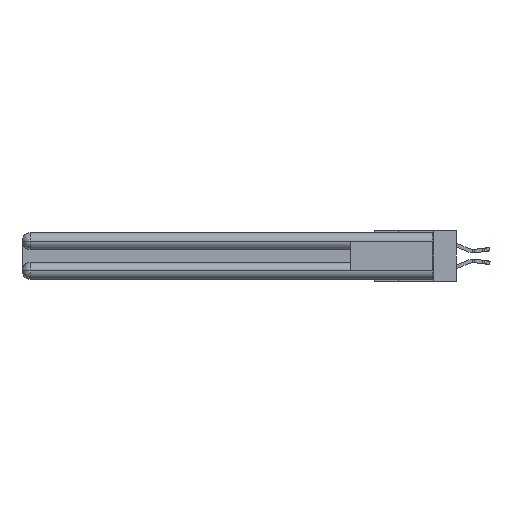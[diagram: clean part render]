
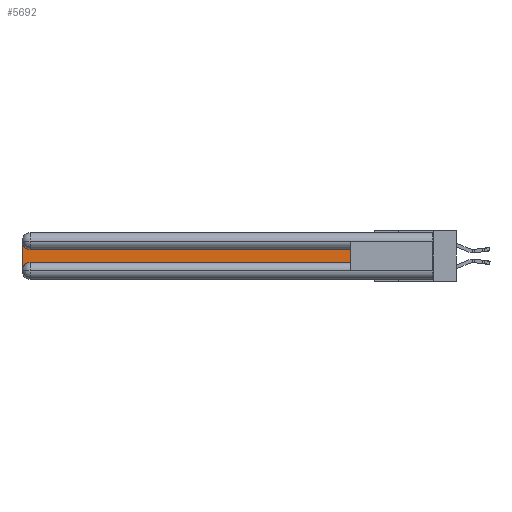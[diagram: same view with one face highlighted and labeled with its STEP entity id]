
A CAD part, left-side view. The second image highlights one B-rep face of the part: STEP entity #5692.
In plain terms, the highlighted planar face has unit normal (-1, 0, 0).
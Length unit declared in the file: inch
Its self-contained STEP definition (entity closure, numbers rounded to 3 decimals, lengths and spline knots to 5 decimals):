
#187 = ORIENTED_EDGE ( 'NONE', *, *, #18927, .T. ) ;
#1337 = VECTOR ( 'NONE', #25625, 39.37008 ) ;
#1376 = CIRCLE ( 'NONE', #27915, 0.06 ) ;
#1756 = AXIS2_PLACEMENT_3D ( 'NONE', #16914, #13825, #24627 ) ;
#2219 = CARTESIAN_POINT ( 'NONE',  ( 0.075, 0.6, -0.2175 ) ) ;
#2345 = CARTESIAN_POINT ( 'NONE',  ( 0.075, 2.94, -0.1225 ) ) ;
#2535 = FACE_OUTER_BOUND ( 'NONE', #12113, .T. ) ;
#2604 = CARTESIAN_POINT ( 'NONE',  ( 0.075, 0.6, -0.1225 ) ) ;
#2699 = VERTEX_POINT ( 'NONE', #16572 ) ;
#3149 = VERTEX_POINT ( 'NONE', #26101 ) ;
#4507 = EDGE_CURVE ( 'NONE', #18697, #16139, #31828, .T. ) ;
#5692 = ADVANCED_FACE ( 'NONE', ( #2535 ), #24978, .F. ) ;
#6351 = CARTESIAN_POINT ( 'NONE',  ( 0.075, 3., -0.0625 ) ) ;
#9904 = CARTESIAN_POINT ( 'NONE',  ( 0.075, 2.94, -0.0625 ) ) ;
#10360 = VERTEX_POINT ( 'NONE', #6351 ) ;
#12113 = EDGE_LOOP ( 'NONE', ( #25393, #34371, #187, #15565, #23285, #22623 ) ) ;
#13825 = DIRECTION ( 'NONE',  ( 1., 0., 0. ) ) ;
#13945 = VERTEX_POINT ( 'NONE', #16155 ) ;
#14497 = LINE ( 'NONE', #17268, #23441 ) ;
#15565 = ORIENTED_EDGE ( 'NONE', *, *, #28559, .T. ) ;
#15616 = DIRECTION ( 'NONE',  ( 1., 0., 0. ) ) ;
#16139 = VERTEX_POINT ( 'NONE', #2345 ) ;
#16155 = CARTESIAN_POINT ( 'NONE',  ( 0.075, 0.6, -0.2175 ) ) ;
#16572 = CARTESIAN_POINT ( 'NONE',  ( 0.075, 2.94, -0.2175 ) ) ;
#16914 = CARTESIAN_POINT ( 'NONE',  ( 0.075, 3., -0.1225 ) ) ;
#17268 = CARTESIAN_POINT ( 'NONE',  ( 0.075, 3., -0.2175 ) ) ;
#17328 = DIRECTION ( 'NONE',  ( 0., 0., 1. ) ) ;
#17354 = CARTESIAN_POINT ( 'NONE',  ( 0.075, 0.6, -0.1225 ) ) ;
#18004 = LINE ( 'NONE', #28317, #20574 ) ;
#18432 = DIRECTION ( 'NONE',  ( 0., 0., -1. ) ) ;
#18697 = VERTEX_POINT ( 'NONE', #2604 ) ;
#18780 = DIRECTION ( 'NONE',  ( 1., 0., 0. ) ) ;
#18927 = EDGE_CURVE ( 'NONE', #10360, #3149, #14497, .T. ) ;
#20356 = LINE ( 'NONE', #2219, #32177 ) ;
#20574 = VECTOR ( 'NONE', #17328, 39.37008 ) ;
#21432 = DIRECTION ( 'NONE',  ( 0., -1., 0. ) ) ;
#21511 = CARTESIAN_POINT ( 'NONE',  ( 0.075, 2.94, -0.2775 ) ) ;
#22623 = ORIENTED_EDGE ( 'NONE', *, *, #29104, .T. ) ;
#23140 = CIRCLE ( 'NONE', #33554, 0.06 ) ;
#23285 = ORIENTED_EDGE ( 'NONE', *, *, #32661, .T. ) ;
#23441 = VECTOR ( 'NONE', #33589, 39.37008 ) ;
#24627 = DIRECTION ( 'NONE',  ( 0., 0., -1. ) ) ;
#24978 = PLANE ( 'NONE',  #1756 ) ;
#25393 = ORIENTED_EDGE ( 'NONE', *, *, #4507, .T. ) ;
#25625 = DIRECTION ( 'NONE',  ( 0., 1., 0. ) ) ;
#26101 = CARTESIAN_POINT ( 'NONE',  ( 0.075, 3., -0.2775 ) ) ;
#27915 = AXIS2_PLACEMENT_3D ( 'NONE', #9904, #15616, #28863 ) ;
#28317 = CARTESIAN_POINT ( 'NONE',  ( 0.075, 0.6, -0.2175 ) ) ;
#28559 = EDGE_CURVE ( 'NONE', #3149, #2699, #23140, .T. ) ;
#28863 = DIRECTION ( 'NONE',  ( 0., 0., -1. ) ) ;
#29104 = EDGE_CURVE ( 'NONE', #13945, #18697, #18004, .T. ) ;
#30460 = EDGE_CURVE ( 'NONE', #16139, #10360, #1376, .T. ) ;
#31828 = LINE ( 'NONE', #17354, #1337 ) ;
#32177 = VECTOR ( 'NONE', #21432, 39.37008 ) ;
#32661 = EDGE_CURVE ( 'NONE', #2699, #13945, #20356, .T. ) ;
#33554 = AXIS2_PLACEMENT_3D ( 'NONE', #21511, #18780, #18432 ) ;
#33589 = DIRECTION ( 'NONE',  ( 0., 0., -1. ) ) ;
#34371 = ORIENTED_EDGE ( 'NONE', *, *, #30460, .T. ) ;
